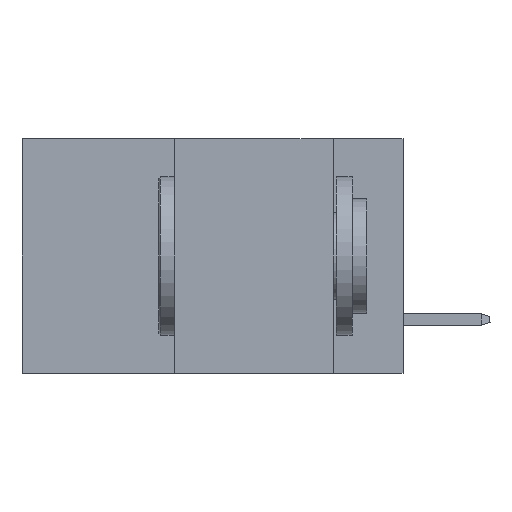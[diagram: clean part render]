
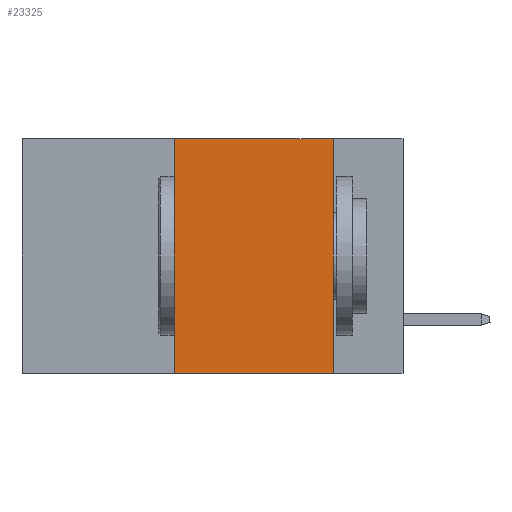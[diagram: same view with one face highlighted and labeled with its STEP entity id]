
A CAD part, left-side view. The second image highlights one B-rep face of the part: STEP entity #23325.
In plain terms, the highlighted planar face has unit normal (-1, 0, 0).
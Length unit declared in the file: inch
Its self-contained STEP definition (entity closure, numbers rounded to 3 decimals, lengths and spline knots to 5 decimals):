
#805 = CARTESIAN_POINT ( 'NONE',  ( 0., 0.36, 0. ) ) ;
#1720 = DIRECTION ( 'NONE',  ( 0., 0., -1. ) ) ;
#2175 = DIRECTION ( 'NONE',  ( 0., -1., 0. ) ) ;
#3656 = VERTEX_POINT ( 'NONE', #28965 ) ;
#5406 = VECTOR ( 'NONE', #23553, 39.37008 ) ;
#5454 = VERTEX_POINT ( 'NONE', #25931 ) ;
#6204 = PLANE ( 'NONE',  #17618 ) ;
#6791 = ORIENTED_EDGE ( 'NONE', *, *, #21296, .F. ) ;
#9895 = DIRECTION ( 'NONE',  ( 0., -1., 0. ) ) ;
#10141 = CARTESIAN_POINT ( 'NONE',  ( 0., 0.6, -0.37 ) ) ;
#12249 = LINE ( 'NONE', #27672, #35375 ) ;
#14108 = ORIENTED_EDGE ( 'NONE', *, *, #28785, .F. ) ;
#14413 = EDGE_LOOP ( 'NONE', ( #46172, #6791, #14108, #15223 ) ) ;
#15223 = ORIENTED_EDGE ( 'NONE', *, *, #39455, .T. ) ;
#17182 = CARTESIAN_POINT ( 'NONE',  ( 0., 0.11, -0.37 ) ) ;
#17618 = AXIS2_PLACEMENT_3D ( 'NONE', #47489, #35795, #1720 ) ;
#21066 = CARTESIAN_POINT ( 'NONE',  ( 0., 0.6, 0. ) ) ;
#21296 = EDGE_CURVE ( 'NONE', #28725, #3656, #39972, .T. ) ;
#23062 = LINE ( 'NONE', #42215, #5406 ) ;
#23325 = ADVANCED_FACE ( 'NONE', ( #25096 ), #6204, .F. ) ;
#23553 = DIRECTION ( 'NONE',  ( 0., 0., -1. ) ) ;
#25096 = FACE_OUTER_BOUND ( 'NONE', #14413, .T. ) ;
#25931 = CARTESIAN_POINT ( 'NONE',  ( 0., 0.36, -0.37 ) ) ;
#27672 = CARTESIAN_POINT ( 'NONE',  ( 0., 0.36, 0. ) ) ;
#28725 = VERTEX_POINT ( 'NONE', #805 ) ;
#28785 = EDGE_CURVE ( 'NONE', #5454, #28725, #12249, .T. ) ;
#28965 = CARTESIAN_POINT ( 'NONE',  ( 0., 0.11, 0. ) ) ;
#35375 = VECTOR ( 'NONE', #42846, 39.37008 ) ;
#35561 = EDGE_CURVE ( 'NONE', #3656, #36761, #23062, .T. ) ;
#35795 = DIRECTION ( 'NONE',  ( 1., 0., 0. ) ) ;
#36761 = VERTEX_POINT ( 'NONE', #17182 ) ;
#38893 = VECTOR ( 'NONE', #2175, 39.37008 ) ;
#39455 = EDGE_CURVE ( 'NONE', #5454, #36761, #47949, .T. ) ;
#39972 = LINE ( 'NONE', #21066, #38893 ) ;
#42175 = VECTOR ( 'NONE', #9895, 39.37008 ) ;
#42215 = CARTESIAN_POINT ( 'NONE',  ( 0., 0.11, 0. ) ) ;
#42846 = DIRECTION ( 'NONE',  ( 0., 0., 1. ) ) ;
#46172 = ORIENTED_EDGE ( 'NONE', *, *, #35561, .F. ) ;
#47489 = CARTESIAN_POINT ( 'NONE',  ( 0., 0.6, 0. ) ) ;
#47949 = LINE ( 'NONE', #10141, #42175 ) ;
